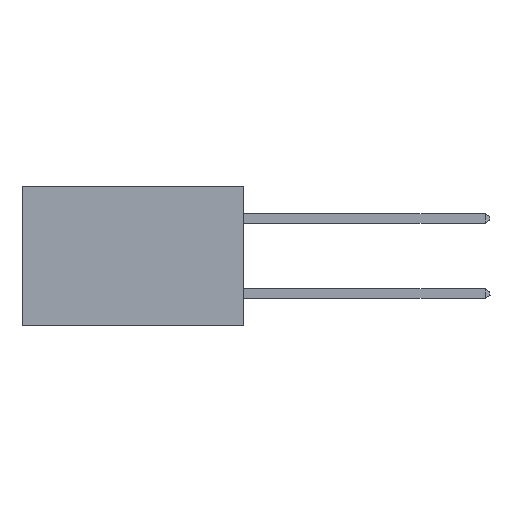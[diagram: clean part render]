
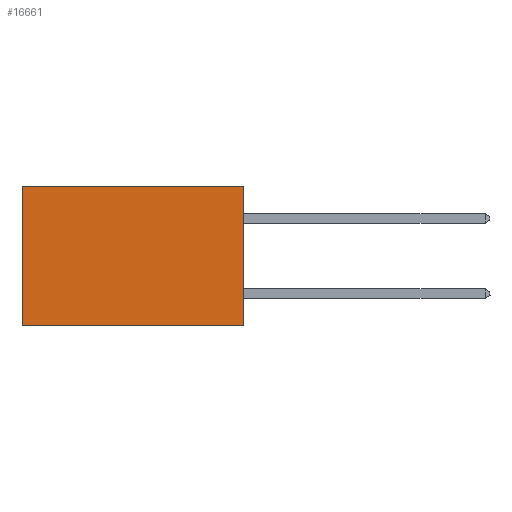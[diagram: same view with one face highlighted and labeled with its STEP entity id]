
A CAD part, left-side view. The second image highlights one B-rep face of the part: STEP entity #16661.
In plain terms, the highlighted planar face has unit normal (-1, 0, 0).
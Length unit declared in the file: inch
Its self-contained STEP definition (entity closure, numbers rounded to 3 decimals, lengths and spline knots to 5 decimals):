
#1640 = CARTESIAN_POINT ( 'NONE',  ( 0.277, 0., -0.37 ) ) ;
#1787 = AXIS2_PLACEMENT_3D ( 'NONE', #26811, #22156, #7910 ) ;
#3174 = VERTEX_POINT ( 'NONE', #5447 ) ;
#4314 = CARTESIAN_POINT ( 'NONE',  ( 0.277, 0.59, -0.37 ) ) ;
#4478 = LINE ( 'NONE', #7848, #28288 ) ;
#4719 = VERTEX_POINT ( 'NONE', #16405 ) ;
#5447 = CARTESIAN_POINT ( 'NONE',  ( 0.277, 0.59, 0. ) ) ;
#7848 = CARTESIAN_POINT ( 'NONE',  ( 0.277, 0., 0. ) ) ;
#7897 = VECTOR ( 'NONE', #11228, 39.37008 ) ;
#7910 = DIRECTION ( 'NONE',  ( 0., 0., -1. ) ) ;
#10001 = EDGE_CURVE ( 'NONE', #4719, #3174, #4478, .T. ) ;
#10857 = ORIENTED_EDGE ( 'NONE', *, *, #26205, .F. ) ;
#11228 = DIRECTION ( 'NONE',  ( 0., 0., -1. ) ) ;
#11717 = VECTOR ( 'NONE', #25227, 39.37008 ) ;
#12698 = DIRECTION ( 'NONE',  ( 0., 0., -1. ) ) ;
#14195 = EDGE_CURVE ( 'NONE', #3174, #21369, #18739, .T. ) ;
#14218 = LINE ( 'NONE', #1640, #7897 ) ;
#15620 = ORIENTED_EDGE ( 'NONE', *, *, #10001, .T. ) ;
#16119 = FACE_OUTER_BOUND ( 'NONE', #25001, .T. ) ;
#16405 = CARTESIAN_POINT ( 'NONE',  ( 0.277, 0., 0. ) ) ;
#16661 = ADVANCED_FACE ( 'NONE', ( #16119 ), #19649, .F. ) ;
#16944 = EDGE_CURVE ( 'NONE', #4719, #17488, #14218, .T. ) ;
#17488 = VERTEX_POINT ( 'NONE', #19804 ) ;
#18054 = LINE ( 'NONE', #18084, #11717 ) ;
#18084 = CARTESIAN_POINT ( 'NONE',  ( 0.277, 0., -0.37 ) ) ;
#18739 = LINE ( 'NONE', #24513, #19471 ) ;
#19172 = ORIENTED_EDGE ( 'NONE', *, *, #14195, .T. ) ;
#19471 = VECTOR ( 'NONE', #12698, 39.37008 ) ;
#19649 = PLANE ( 'NONE',  #1787 ) ;
#19804 = CARTESIAN_POINT ( 'NONE',  ( 0.277, 0., -0.37 ) ) ;
#21369 = VERTEX_POINT ( 'NONE', #4314 ) ;
#22156 = DIRECTION ( 'NONE',  ( 1., 0., 0. ) ) ;
#24513 = CARTESIAN_POINT ( 'NONE',  ( 0.277, 0.59, -0.37 ) ) ;
#25001 = EDGE_LOOP ( 'NONE', ( #19172, #10857, #30130, #15620 ) ) ;
#25227 = DIRECTION ( 'NONE',  ( 0., 1., 0. ) ) ;
#26205 = EDGE_CURVE ( 'NONE', #17488, #21369, #18054, .T. ) ;
#26811 = CARTESIAN_POINT ( 'NONE',  ( 0.277, 0., -0.37 ) ) ;
#26864 = DIRECTION ( 'NONE',  ( 0., 1., 0. ) ) ;
#28288 = VECTOR ( 'NONE', #26864, 39.37008 ) ;
#30130 = ORIENTED_EDGE ( 'NONE', *, *, #16944, .F. ) ;
